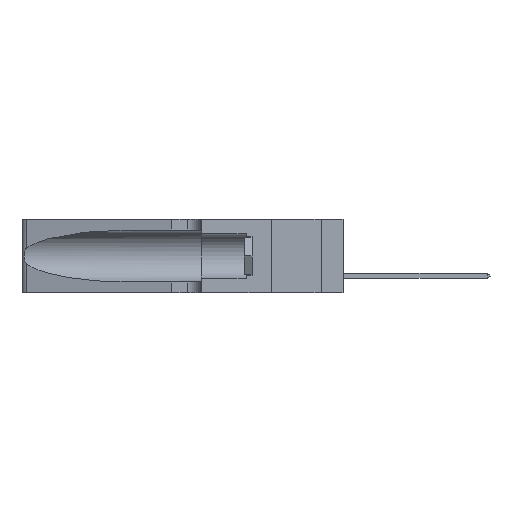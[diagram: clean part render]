
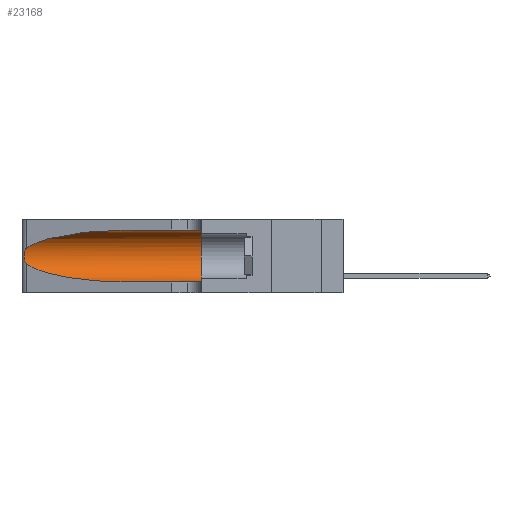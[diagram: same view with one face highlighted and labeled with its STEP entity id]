
A CAD part, left-side view. The second image highlights one B-rep face of the part: STEP entity #23168.
In plain terms, the highlighted cylindrical face has radius 3.308 mm (diameter 6.617 mm), a partial arc.
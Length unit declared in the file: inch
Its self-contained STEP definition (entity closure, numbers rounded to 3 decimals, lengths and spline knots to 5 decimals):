
#1185 = DIRECTION ( 'NONE',  ( 0., -1., 0. ) ) ;
#1475 = EDGE_CURVE ( 'NONE', #9243, #22811, #8038, .T. ) ;
#3318 = CARTESIAN_POINT ( 'NONE',  ( 0.2373, 1.15595, 0.28018 ) ) ;
#4093 = EDGE_LOOP ( 'NONE', ( #16472, #19844, #38178, #36629, #39748, #32617 ) ) ;
#4876 = DIRECTION ( 'NONE',  ( 0., -1., 0. ) ) ;
#4910 =( BOUNDED_CURVE ( )  B_SPLINE_CURVE ( 3, ( #19623, #6473, #27149, #20045 ),
 .UNSPECIFIED., .F., .F. ) 
 B_SPLINE_CURVE_WITH_KNOTS ( ( 4, 4 ),
 ( 3.44316, 4.71239 ),
 .UNSPECIFIED. ) 
 CURVE ( )  GEOMETRIC_REPRESENTATION_ITEM ( )  RATIONAL_B_SPLINE_CURVE ( ( 1., 0.87, 0.87, 1. ) ) 
 REPRESENTATION_ITEM ( '' )  );
#5057 = CARTESIAN_POINT ( 'NONE',  ( 0.25787, 1.23484, 0.2124 ) ) ;
#5198 = CARTESIAN_POINT ( 'NONE',  ( 0.25487, 1.22718, 0.14631 ) ) ;
#6322 = CARTESIAN_POINT ( 'NONE',  ( 0.1305, 0.72297, 0.31525 ) ) ;
#6450 = CYLINDRICAL_SURFACE ( 'NONE', #33268, 0.13025 ) ;
#6473 = CARTESIAN_POINT ( 'NONE',  ( 0.2373, 1.15595, 0.08982 ) ) ;
#6746 = CARTESIAN_POINT ( 'NONE',  ( 0.25487, 1.22718, 0.22369 ) ) ;
#7094 = CARTESIAN_POINT ( 'NONE',  ( 0.1305, 0.35, 0.31525 ) ) ;
#7185 = VERTEX_POINT ( 'NONE', #34267 ) ;
#7643 = CARTESIAN_POINT ( 'NONE',  ( 0.25487, 1.22718, 0.22369 ) ) ;
#7902 = CARTESIAN_POINT ( 'NONE',  ( 0.25487, 1.22718, 0.22369 ) ) ;
#8038 =( BOUNDED_CURVE ( )  B_SPLINE_CURVE ( 3, ( #6322, #22898, #3318, #6746 ),
 .UNSPECIFIED., .F., .T. ) 
 B_SPLINE_CURVE_WITH_KNOTS ( ( 4, 4 ),
 ( 1.5708, 2.84003 ),
 .UNSPECIFIED. ) 
 CURVE ( )  GEOMETRIC_REPRESENTATION_ITEM ( )  RATIONAL_B_SPLINE_CURVE ( ( 1., 0.87, 0.87, 1. ) ) 
 REPRESENTATION_ITEM ( '' )  );
#8149 = CARTESIAN_POINT ( 'NONE',  ( 0.1305, 1.61858, 0.31525 ) ) ;
#8323 = CARTESIAN_POINT ( 'NONE',  ( 0.25854, 1.2359, 0.20912 ) ) ;
#9243 = VERTEX_POINT ( 'NONE', #36907 ) ;
#10880 = LINE ( 'NONE', #17244, #25072 ) ;
#11607 = CARTESIAN_POINT ( 'NONE',  ( 0.26075, 1.23896, 0.178 ) ) ;
#11864 = AXIS2_PLACEMENT_3D ( 'NONE', #39907, #23508, #27198 ) ;
#13155 = EDGE_CURVE ( 'NONE', #29375, #7185, #16945, .T. ) ;
#13167 = EDGE_CURVE ( 'NONE', #26775, #7185, #10880, .T. ) ;
#14820 = CARTESIAN_POINT ( 'NONE',  ( 0.25856, 1.23593, 0.16098 ) ) ;
#16472 = ORIENTED_EDGE ( 'NONE', *, *, #1475, .T. ) ;
#16945 = CIRCLE ( 'NONE', #11864, 0.13025 ) ;
#16952 = VERTEX_POINT ( 'NONE', #18672 ) ;
#16965 = DIRECTION ( 'NONE',  ( 0., -1., 0. ) ) ;
#17074 = CARTESIAN_POINT ( 'NONE',  ( 0.1305, 1.61858, 0.185 ) ) ;
#17244 = CARTESIAN_POINT ( 'NONE',  ( 0.1305, 1.61858, 0.05475 ) ) ;
#17688 = CARTESIAN_POINT ( 'NONE',  ( 0.26018, 1.23835, 0.19895 ) ) ;
#18672 = CARTESIAN_POINT ( 'NONE',  ( 0.25487, 1.22718, 0.14631 ) ) ;
#19331 = VECTOR ( 'NONE', #4876, 39.37008 ) ;
#19623 = CARTESIAN_POINT ( 'NONE',  ( 0.25487, 1.22718, 0.14631 ) ) ;
#19844 = ORIENTED_EDGE ( 'NONE', *, *, #33480, .T. ) ;
#20045 = CARTESIAN_POINT ( 'NONE',  ( 0.1305, 0.72297, 0.05475 ) ) ;
#20942 = CARTESIAN_POINT ( 'NONE',  ( 0.25789, 1.23486, 0.15765 ) ) ;
#21467 = EDGE_CURVE ( 'NONE', #16952, #26775, #4910, .T. ) ;
#22811 = VERTEX_POINT ( 'NONE', #7643 ) ;
#22898 = CARTESIAN_POINT ( 'NONE',  ( 0.18966, 0.96281, 0.31525 ) ) ;
#23168 = ADVANCED_FACE ( 'NONE', ( #36850 ), #6450, .F. ) ;
#23508 = DIRECTION ( 'NONE',  ( 0., 1., 0. ) ) ;
#24206 = CARTESIAN_POINT ( 'NONE',  ( 0.25639, 1.23186, 0.15144 ) ) ;
#25072 = VECTOR ( 'NONE', #16965, 39.37008 ) ;
#25825 = CARTESIAN_POINT ( 'NONE',  ( 0.1305, 0.72297, 0.05475 ) ) ;
#26775 = VERTEX_POINT ( 'NONE', #25825 ) ;
#27149 = CARTESIAN_POINT ( 'NONE',  ( 0.18966, 0.96281, 0.05475 ) ) ;
#27198 = DIRECTION ( 'NONE',  ( 0., 0., 1. ) ) ;
#27495 = CARTESIAN_POINT ( 'NONE',  ( 0.25555, 1.22993, 0.14849 ) ) ;
#29375 = VERTEX_POINT ( 'NONE', #7094 ) ;
#29880 = EDGE_CURVE ( 'NONE', #9243, #29375, #37076, .T. ) ;
#31043 = CARTESIAN_POINT ( 'NONE',  ( 0.26075, 1.23896, 0.19203 ) ) ;
#32617 = ORIENTED_EDGE ( 'NONE', *, *, #29880, .F. ) ;
#33059 = B_SPLINE_CURVE_WITH_KNOTS ( 'NONE', 3,
 ( #7902, #37104, #40599, #5057, #8323, #17688, #31043, #11607, #34313, #14820, #20942, #24206, #27495, #5198 ),
 .UNSPECIFIED., .F., .F.,
 ( 4, 2, 2, 2, 2, 2, 4 ),
 ( 0., 0.00027, 0.00053, 0.00107, 0.0016, 0.00187, 0.00214 ),
 .UNSPECIFIED. ) ;
#33268 = AXIS2_PLACEMENT_3D ( 'NONE', #17074, #1185, #33591 ) ;
#33480 = EDGE_CURVE ( 'NONE', #22811, #16952, #33059, .T. ) ;
#33591 = DIRECTION ( 'NONE',  ( 0., 0., -1. ) ) ;
#34267 = CARTESIAN_POINT ( 'NONE',  ( 0.1305, 0.35, 0.05475 ) ) ;
#34313 = CARTESIAN_POINT ( 'NONE',  ( 0.26017, 1.23833, 0.17102 ) ) ;
#36629 = ORIENTED_EDGE ( 'NONE', *, *, #13167, .T. ) ;
#36850 = FACE_OUTER_BOUND ( 'NONE', #4093, .T. ) ;
#36907 = CARTESIAN_POINT ( 'NONE',  ( 0.1305, 0.72297, 0.31525 ) ) ;
#37076 = LINE ( 'NONE', #8149, #19331 ) ;
#37104 = CARTESIAN_POINT ( 'NONE',  ( 0.25555, 1.22994, 0.2215 ) ) ;
#38178 = ORIENTED_EDGE ( 'NONE', *, *, #21467, .T. ) ;
#39748 = ORIENTED_EDGE ( 'NONE', *, *, #13155, .F. ) ;
#39907 = CARTESIAN_POINT ( 'NONE',  ( 0.1305, 0.35, 0.185 ) ) ;
#40599 = CARTESIAN_POINT ( 'NONE',  ( 0.25639, 1.23184, 0.21858 ) ) ;
